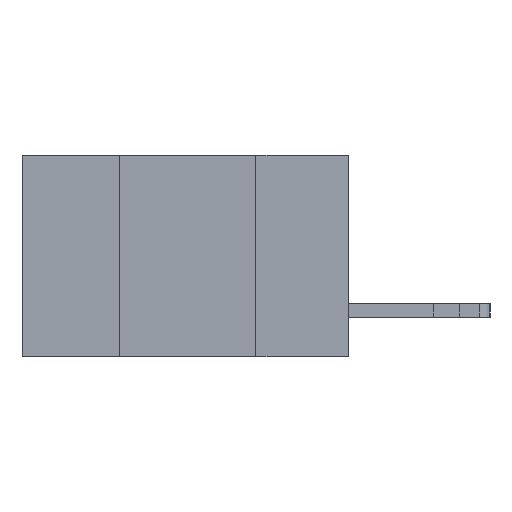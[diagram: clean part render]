
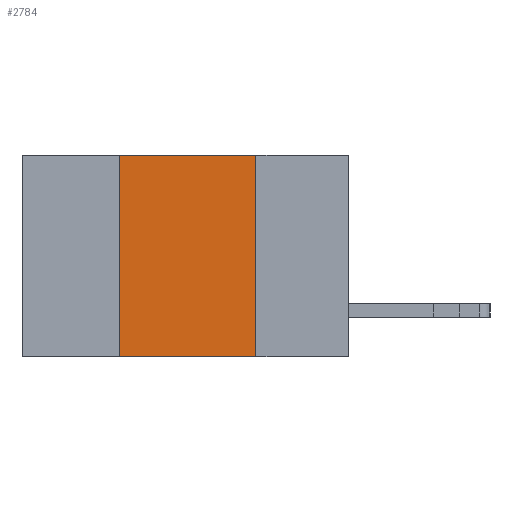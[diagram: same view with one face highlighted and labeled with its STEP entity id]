
A CAD part, left-side view. The second image highlights one B-rep face of the part: STEP entity #2784.
In plain terms, the highlighted planar face has unit normal (-1, 0, 0).
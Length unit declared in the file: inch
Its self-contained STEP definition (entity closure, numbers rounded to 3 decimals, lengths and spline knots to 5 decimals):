
#490 = EDGE_CURVE ( 'NONE', #1010, #7774, #5426, .T. ) ;
#939 = DIRECTION ( 'NONE',  ( 0., -1., 0. ) ) ;
#1010 = VERTEX_POINT ( 'NONE', #1043 ) ;
#1043 = CARTESIAN_POINT ( 'NONE',  ( 0., 0.42, 0. ) ) ;
#2524 = EDGE_CURVE ( 'NONE', #5451, #2980, #5976, .T. ) ;
#2721 = CARTESIAN_POINT ( 'NONE',  ( 0., 0.17, -0.37 ) ) ;
#2784 = ADVANCED_FACE ( 'NONE', ( #4307 ), #5406, .F. ) ;
#2926 = ORIENTED_EDGE ( 'NONE', *, *, #6907, .F. ) ;
#2980 = VERTEX_POINT ( 'NONE', #2721 ) ;
#3176 = VECTOR ( 'NONE', #4533, 39.37008 ) ;
#3533 = VECTOR ( 'NONE', #939, 39.37008 ) ;
#3816 = CARTESIAN_POINT ( 'NONE',  ( 0., 0.42, -0.37 ) ) ;
#4307 = FACE_OUTER_BOUND ( 'NONE', #4642, .T. ) ;
#4457 = CARTESIAN_POINT ( 'NONE',  ( 0., 0.17, 0. ) ) ;
#4533 = DIRECTION ( 'NONE',  ( 0., 0., 1. ) ) ;
#4642 = EDGE_LOOP ( 'NONE', ( #2926, #8116, #7863, #5004 ) ) ;
#5004 = ORIENTED_EDGE ( 'NONE', *, *, #2524, .T. ) ;
#5121 = LINE ( 'NONE', #3816, #3176 ) ;
#5253 = DIRECTION ( 'NONE',  ( 1., 0., 0. ) ) ;
#5347 = CARTESIAN_POINT ( 'NONE',  ( 0., 0.6, 0. ) ) ;
#5406 = PLANE ( 'NONE',  #5853 ) ;
#5426 = LINE ( 'NONE', #8898, #3533 ) ;
#5451 = VERTEX_POINT ( 'NONE', #8743 ) ;
#5538 = VECTOR ( 'NONE', #8662, 39.37008 ) ;
#5565 = VECTOR ( 'NONE', #6560, 39.37008 ) ;
#5853 = AXIS2_PLACEMENT_3D ( 'NONE', #5347, #5253, #6824 ) ;
#5976 = LINE ( 'NONE', #8641, #5538 ) ;
#6560 = DIRECTION ( 'NONE',  ( 0., 0., -1. ) ) ;
#6587 = CARTESIAN_POINT ( 'NONE',  ( 0., 0.17, -0.37 ) ) ;
#6824 = DIRECTION ( 'NONE',  ( 0., 0., -1. ) ) ;
#6907 = EDGE_CURVE ( 'NONE', #7774, #2980, #9365, .T. ) ;
#6967 = EDGE_CURVE ( 'NONE', #5451, #1010, #5121, .T. ) ;
#7774 = VERTEX_POINT ( 'NONE', #4457 ) ;
#7863 = ORIENTED_EDGE ( 'NONE', *, *, #6967, .F. ) ;
#8116 = ORIENTED_EDGE ( 'NONE', *, *, #490, .F. ) ;
#8641 = CARTESIAN_POINT ( 'NONE',  ( 0., 0.6, -0.37 ) ) ;
#8662 = DIRECTION ( 'NONE',  ( 0., -1., 0. ) ) ;
#8743 = CARTESIAN_POINT ( 'NONE',  ( 0., 0.42, -0.37 ) ) ;
#8898 = CARTESIAN_POINT ( 'NONE',  ( 0., 0.6, 0. ) ) ;
#9365 = LINE ( 'NONE', #6587, #5565 ) ;
